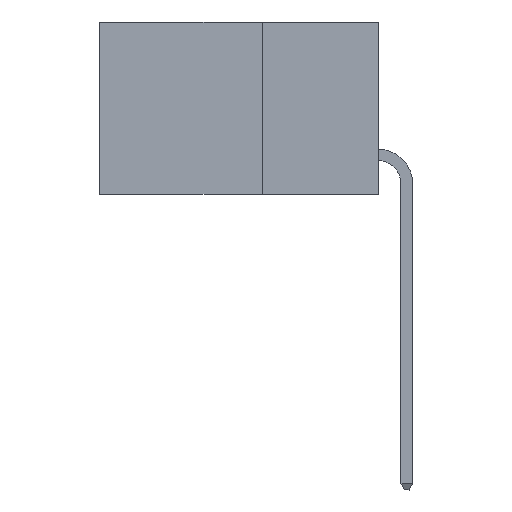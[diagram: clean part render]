
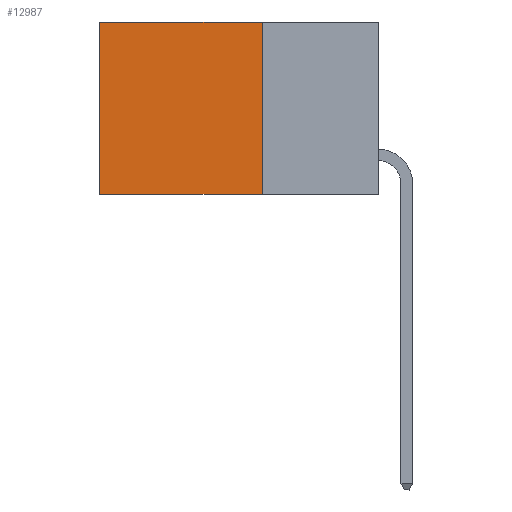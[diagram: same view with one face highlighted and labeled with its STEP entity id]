
A CAD part, left-side view. The second image highlights one B-rep face of the part: STEP entity #12987.
In plain terms, the highlighted planar face has unit normal (-1, 0, 0).
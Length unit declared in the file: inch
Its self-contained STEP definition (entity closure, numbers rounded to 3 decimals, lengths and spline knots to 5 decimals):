
#55 = DIRECTION ( 'NONE',  ( 0., 0., -1. ) ) ;
#747 = EDGE_LOOP ( 'NONE', ( #15959, #6295, #6606, #12927 ) ) ;
#808 = FACE_OUTER_BOUND ( 'NONE', #747, .T. ) ;
#1570 = LINE ( 'NONE', #6045, #13717 ) ;
#2564 = CARTESIAN_POINT ( 'NONE',  ( 0.2615, 0.6, -0.37 ) ) ;
#2780 = EDGE_CURVE ( 'NONE', #11902, #5802, #8298, .T. ) ;
#3690 = EDGE_CURVE ( 'NONE', #5802, #9591, #16729, .T. ) ;
#5349 = DIRECTION ( 'NONE',  ( 0., 0., -1. ) ) ;
#5576 = CARTESIAN_POINT ( 'NONE',  ( 0.2615, 0.25, 0. ) ) ;
#5588 = CARTESIAN_POINT ( 'NONE',  ( 0.2615, 0.6, 0. ) ) ;
#5759 = CARTESIAN_POINT ( 'NONE',  ( 0.2615, 0.25, -0.37 ) ) ;
#5802 = VERTEX_POINT ( 'NONE', #5588 ) ;
#5921 = CARTESIAN_POINT ( 'NONE',  ( 0.2615, 0.25, -0.37 ) ) ;
#6045 = CARTESIAN_POINT ( 'NONE',  ( 0.2615, 0.25, -0.37 ) ) ;
#6087 = CARTESIAN_POINT ( 'NONE',  ( 0.2615, 0.25, 0. ) ) ;
#6238 = EDGE_CURVE ( 'NONE', #11902, #18415, #15707, .T. ) ;
#6295 = ORIENTED_EDGE ( 'NONE', *, *, #7095, .F. ) ;
#6521 = PLANE ( 'NONE',  #16519 ) ;
#6606 = ORIENTED_EDGE ( 'NONE', *, *, #6238, .F. ) ;
#7095 = EDGE_CURVE ( 'NONE', #18415, #9591, #1570, .T. ) ;
#7177 = DIRECTION ( 'NONE',  ( 1., 0., 0. ) ) ;
#7437 = VECTOR ( 'NONE', #5349, 39.37008 ) ;
#8298 = LINE ( 'NONE', #5576, #8966 ) ;
#8456 = CARTESIAN_POINT ( 'NONE',  ( 0.2615, 0.6, -0.37 ) ) ;
#8966 = VECTOR ( 'NONE', #11237, 39.37008 ) ;
#9591 = VERTEX_POINT ( 'NONE', #2564 ) ;
#9905 = DIRECTION ( 'NONE',  ( 0., 0., -1. ) ) ;
#11237 = DIRECTION ( 'NONE',  ( 0., 1., 0. ) ) ;
#11805 = DIRECTION ( 'NONE',  ( 0., 1., 0. ) ) ;
#11902 = VERTEX_POINT ( 'NONE', #6087 ) ;
#12927 = ORIENTED_EDGE ( 'NONE', *, *, #2780, .T. ) ;
#12987 = ADVANCED_FACE ( 'NONE', ( #808 ), #6521, .F. ) ;
#13465 = VECTOR ( 'NONE', #9905, 39.37008 ) ;
#13717 = VECTOR ( 'NONE', #11805, 39.37008 ) ;
#13947 = CARTESIAN_POINT ( 'NONE',  ( 0.2615, 0.25, -0.37 ) ) ;
#15707 = LINE ( 'NONE', #5921, #13465 ) ;
#15959 = ORIENTED_EDGE ( 'NONE', *, *, #3690, .T. ) ;
#16519 = AXIS2_PLACEMENT_3D ( 'NONE', #5759, #7177, #55 ) ;
#16729 = LINE ( 'NONE', #8456, #7437 ) ;
#18415 = VERTEX_POINT ( 'NONE', #13947 ) ;
